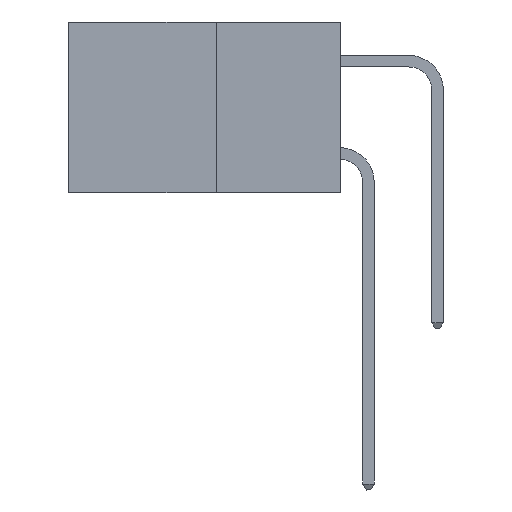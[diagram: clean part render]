
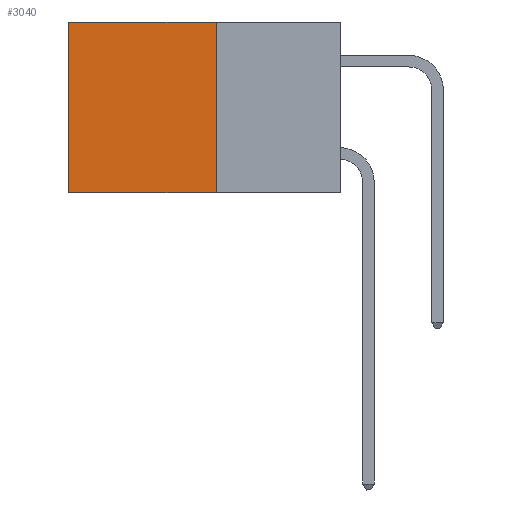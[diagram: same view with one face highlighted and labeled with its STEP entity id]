
A CAD part, left-side view. The second image highlights one B-rep face of the part: STEP entity #3040.
In plain terms, the highlighted planar face has unit normal (-1, 0, 0).
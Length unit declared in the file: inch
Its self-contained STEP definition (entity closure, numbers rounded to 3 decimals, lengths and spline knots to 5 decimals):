
#394 = DIRECTION ( 'NONE',  ( 0., 0., -1. ) ) ;
#1939 = EDGE_CURVE ( 'NONE', #15673, #5651, #13665, .T. ) ;
#3040 = ADVANCED_FACE ( 'NONE', ( #18680 ), #16222, .F. ) ;
#3488 = DIRECTION ( 'NONE',  ( 0., 1., 0. ) ) ;
#4349 = VECTOR ( 'NONE', #21780, 39.37008 ) ;
#4980 = ORIENTED_EDGE ( 'NONE', *, *, #6004, .F. ) ;
#5023 = EDGE_CURVE ( 'NONE', #16062, #15673, #5370, .T. ) ;
#5370 = LINE ( 'NONE', #12756, #19415 ) ;
#5651 = VERTEX_POINT ( 'NONE', #21636 ) ;
#6004 = EDGE_CURVE ( 'NONE', #14789, #5651, #9118, .T. ) ;
#6235 = ORIENTED_EDGE ( 'NONE', *, *, #1939, .T. ) ;
#8651 = VECTOR ( 'NONE', #394, 39.37008 ) ;
#9118 = LINE ( 'NONE', #13528, #18255 ) ;
#10758 = DIRECTION ( 'NONE',  ( 0., 0., -1. ) ) ;
#11027 = ORIENTED_EDGE ( 'NONE', *, *, #5023, .T. ) ;
#11042 = DIRECTION ( 'NONE',  ( 1., 0., 0. ) ) ;
#11508 = CARTESIAN_POINT ( 'NONE',  ( 0.277, 0.27, -0.37 ) ) ;
#12756 = CARTESIAN_POINT ( 'NONE',  ( 0.277, 0.27, 0. ) ) ;
#13195 = AXIS2_PLACEMENT_3D ( 'NONE', #15630, #11042, #10758 ) ;
#13528 = CARTESIAN_POINT ( 'NONE',  ( 0.277, 0.27, -0.37 ) ) ;
#13665 = LINE ( 'NONE', #21871, #4349 ) ;
#14062 = CARTESIAN_POINT ( 'NONE',  ( 0.277, 0.27, -0.37 ) ) ;
#14329 = CARTESIAN_POINT ( 'NONE',  ( 0.277, 0.27, 0. ) ) ;
#14789 = VERTEX_POINT ( 'NONE', #14062 ) ;
#15354 = DIRECTION ( 'NONE',  ( 0., 1., 0. ) ) ;
#15630 = CARTESIAN_POINT ( 'NONE',  ( 0.277, 0.27, -0.37 ) ) ;
#15673 = VERTEX_POINT ( 'NONE', #20130 ) ;
#16062 = VERTEX_POINT ( 'NONE', #14329 ) ;
#16222 = PLANE ( 'NONE',  #13195 ) ;
#17915 = EDGE_CURVE ( 'NONE', #16062, #14789, #22578, .T. ) ;
#18255 = VECTOR ( 'NONE', #15354, 39.37008 ) ;
#18469 = ORIENTED_EDGE ( 'NONE', *, *, #17915, .F. ) ;
#18680 = FACE_OUTER_BOUND ( 'NONE', #21063, .T. ) ;
#19415 = VECTOR ( 'NONE', #3488, 39.37008 ) ;
#20130 = CARTESIAN_POINT ( 'NONE',  ( 0.277, 0.59, 0. ) ) ;
#21063 = EDGE_LOOP ( 'NONE', ( #6235, #4980, #18469, #11027 ) ) ;
#21636 = CARTESIAN_POINT ( 'NONE',  ( 0.277, 0.59, -0.37 ) ) ;
#21780 = DIRECTION ( 'NONE',  ( 0., 0., -1. ) ) ;
#21871 = CARTESIAN_POINT ( 'NONE',  ( 0.277, 0.59, -0.37 ) ) ;
#22578 = LINE ( 'NONE', #11508, #8651 ) ;
